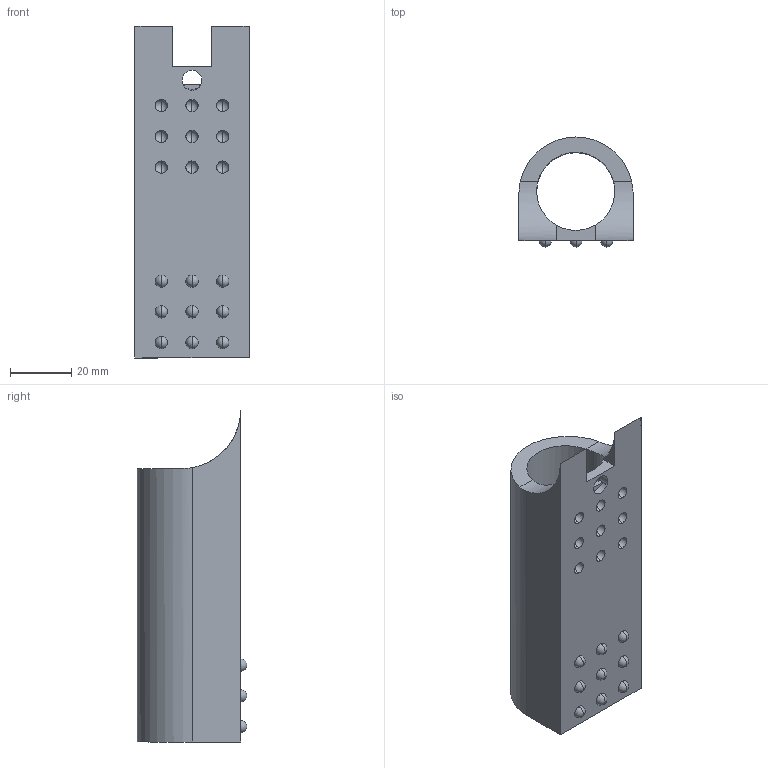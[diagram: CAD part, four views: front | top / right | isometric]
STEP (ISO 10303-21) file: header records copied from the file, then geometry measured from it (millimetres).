
FILE_DESCRIPTION (( 'STEP AP214' ), '1' );
FILE_NAME ('Buffer_Tube_1a_1.step', '2019-12-18T03:07:10', ( '' ), ( '' ), 'SwSTEP 2.0', 'SolidWorks 2019', '' );
FILE_SCHEMA (( 'AUTOMOTIVE_DESIGN' ));
Length unit declared in the file: millimetre
Products named in the file (1): Buffer_Tube_1a_1
Bounding box: 37.13 x 35.66 x 108 mm (x, y, z)
Volume: 54857.5 mm3; surface area: 20851.5 mm2
Topology: 1 solids, 1 shells, 54 faces, 193 edges, 122 vertices
Faces by surface type: sphere 36, plane 10, cylinder 6, bspline 2
Entity records: 1696 total; most frequent: CARTESIAN_POINT 382, DIRECTION 296, ORIENTED_EDGE 242, AXIS2_PLACEMENT_3D 136, EDGE_CURVE 121, VERTEX_POINT 86, CIRCLE 83, EDGE_LOOP 75
